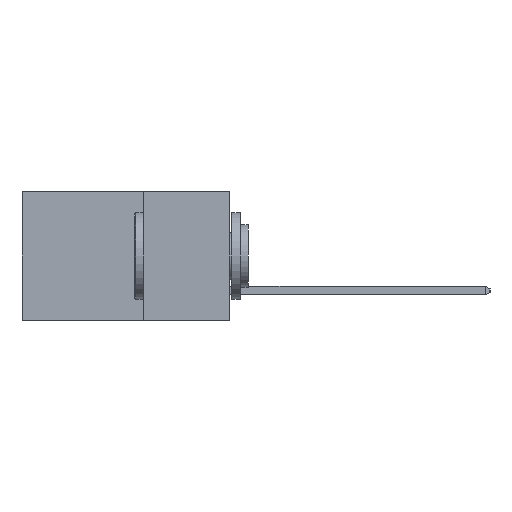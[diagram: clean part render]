
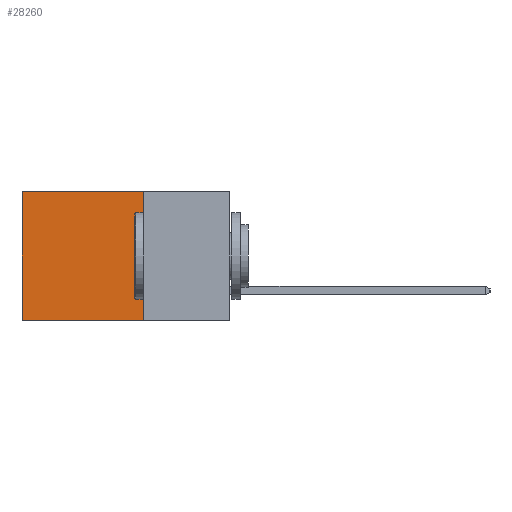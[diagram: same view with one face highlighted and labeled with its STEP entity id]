
A CAD part, left-side view. The second image highlights one B-rep face of the part: STEP entity #28260.
In plain terms, the highlighted planar face has unit normal (-1, 0, 0).
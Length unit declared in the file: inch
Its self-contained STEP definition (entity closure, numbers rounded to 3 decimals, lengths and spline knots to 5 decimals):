
#611 = ORIENTED_EDGE ( 'NONE', *, *, #18826, .F. ) ;
#749 = DIRECTION ( 'NONE',  ( 0., 0., -1. ) ) ;
#1524 = CARTESIAN_POINT ( 'NONE',  ( 0.298, 0.25, -0.37 ) ) ;
#2930 = LINE ( 'NONE', #14238, #14886 ) ;
#6186 = CARTESIAN_POINT ( 'NONE',  ( 0.298, 0.25, 0. ) ) ;
#6194 = VERTEX_POINT ( 'NONE', #22354 ) ;
#6366 = LINE ( 'NONE', #1524, #16179 ) ;
#6662 = DIRECTION ( 'NONE',  ( 0., 0., -1. ) ) ;
#6803 = VECTOR ( 'NONE', #17549, 39.37008 ) ;
#7045 = ORIENTED_EDGE ( 'NONE', *, *, #27804, .T. ) ;
#8771 = EDGE_CURVE ( 'NONE', #6194, #20271, #16594, .T. ) ;
#8883 = FACE_OUTER_BOUND ( 'NONE', #19310, .T. ) ;
#11318 = VECTOR ( 'NONE', #21685, 39.37008 ) ;
#11640 = EDGE_CURVE ( 'NONE', #6194, #24342, #24384, .T. ) ;
#14238 = CARTESIAN_POINT ( 'NONE',  ( 0.298, 0.6, 0. ) ) ;
#14886 = VECTOR ( 'NONE', #749, 39.37008 ) ;
#15239 = CARTESIAN_POINT ( 'NONE',  ( 0.298, 0.25, 0. ) ) ;
#16179 = VECTOR ( 'NONE', #23729, 39.37008 ) ;
#16594 = LINE ( 'NONE', #6186, #11318 ) ;
#17549 = DIRECTION ( 'NONE',  ( 0., 0., -1. ) ) ;
#17709 = ORIENTED_EDGE ( 'NONE', *, *, #8771, .T. ) ;
#17799 = CARTESIAN_POINT ( 'NONE',  ( 0.298, 0.25, 0. ) ) ;
#17976 = AXIS2_PLACEMENT_3D ( 'NONE', #17799, #19996, #6662 ) ;
#18826 = EDGE_CURVE ( 'NONE', #24342, #20471, #6366, .T. ) ;
#19310 = EDGE_LOOP ( 'NONE', ( #7045, #611, #24841, #17709 ) ) ;
#19996 = DIRECTION ( 'NONE',  ( 1., 0., 0. ) ) ;
#20271 = VERTEX_POINT ( 'NONE', #26147 ) ;
#20471 = VERTEX_POINT ( 'NONE', #20508 ) ;
#20508 = CARTESIAN_POINT ( 'NONE',  ( 0.298, 0.6, -0.37 ) ) ;
#21685 = DIRECTION ( 'NONE',  ( 0., 1., 0. ) ) ;
#22354 = CARTESIAN_POINT ( 'NONE',  ( 0.298, 0.25, 0. ) ) ;
#23729 = DIRECTION ( 'NONE',  ( 0., 1., 0. ) ) ;
#24342 = VERTEX_POINT ( 'NONE', #24395 ) ;
#24384 = LINE ( 'NONE', #15239, #6803 ) ;
#24395 = CARTESIAN_POINT ( 'NONE',  ( 0.298, 0.25, -0.37 ) ) ;
#24841 = ORIENTED_EDGE ( 'NONE', *, *, #11640, .F. ) ;
#26147 = CARTESIAN_POINT ( 'NONE',  ( 0.298, 0.6, 0. ) ) ;
#27804 = EDGE_CURVE ( 'NONE', #20271, #20471, #2930, .T. ) ;
#28260 = ADVANCED_FACE ( 'NONE', ( #8883 ), #28513, .F. ) ;
#28513 = PLANE ( 'NONE',  #17976 ) ;
